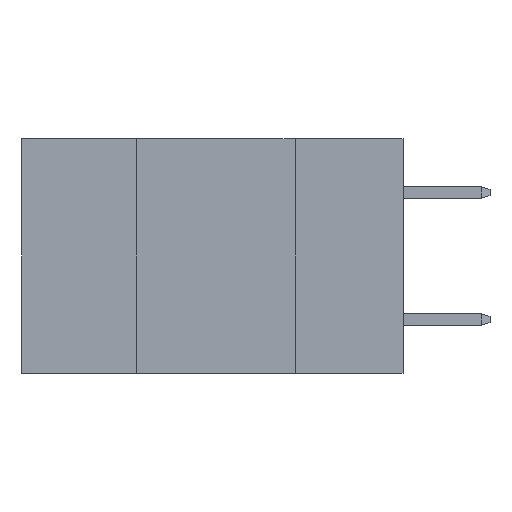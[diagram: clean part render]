
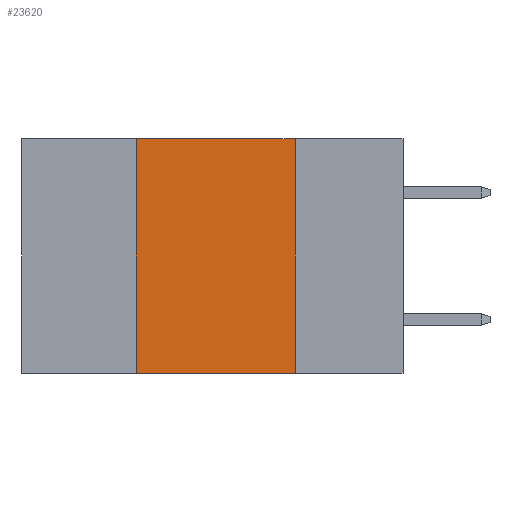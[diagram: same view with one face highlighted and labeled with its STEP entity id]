
A CAD part, left-side view. The second image highlights one B-rep face of the part: STEP entity #23620.
In plain terms, the highlighted planar face has unit normal (-1, 0, 0).
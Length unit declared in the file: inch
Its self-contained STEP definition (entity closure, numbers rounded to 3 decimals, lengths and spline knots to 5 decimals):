
#1171 = DIRECTION ( 'NONE',  ( 0., 0., -1. ) ) ;
#1890 = CARTESIAN_POINT ( 'NONE',  ( 0., 0.17, 0. ) ) ;
#1953 = CARTESIAN_POINT ( 'NONE',  ( 0., 0.6, 0. ) ) ;
#2486 = EDGE_CURVE ( 'NONE', #7120, #14501, #8160, .T. ) ;
#3220 = LINE ( 'NONE', #17928, #13040 ) ;
#3814 = CARTESIAN_POINT ( 'NONE',  ( 0., 0.42, 0. ) ) ;
#4057 = DIRECTION ( 'NONE',  ( 0., -1., 0. ) ) ;
#4792 = PLANE ( 'NONE',  #8637 ) ;
#4900 = CARTESIAN_POINT ( 'NONE',  ( 0., 0.6, 0. ) ) ;
#5756 = LINE ( 'NONE', #1890, #13366 ) ;
#6649 = EDGE_LOOP ( 'NONE', ( #21218, #14954, #16603, #20751 ) ) ;
#7120 = VERTEX_POINT ( 'NONE', #22613 ) ;
#8160 = LINE ( 'NONE', #10052, #16200 ) ;
#8206 = EDGE_CURVE ( 'NONE', #14170, #14501, #5756, .T. ) ;
#8637 = AXIS2_PLACEMENT_3D ( 'NONE', #4900, #18247, #1171 ) ;
#10052 = CARTESIAN_POINT ( 'NONE',  ( 0., 0.6, -0.37 ) ) ;
#10071 = CARTESIAN_POINT ( 'NONE',  ( 0., 0.17, -0.37 ) ) ;
#10818 = EDGE_CURVE ( 'NONE', #7120, #22752, #3220, .T. ) ;
#11164 = DIRECTION ( 'NONE',  ( 0., 0., -1. ) ) ;
#13040 = VECTOR ( 'NONE', #23907, 39.37008 ) ;
#13366 = VECTOR ( 'NONE', #11164, 39.37008 ) ;
#14170 = VERTEX_POINT ( 'NONE', #23656 ) ;
#14501 = VERTEX_POINT ( 'NONE', #10071 ) ;
#14954 = ORIENTED_EDGE ( 'NONE', *, *, #24196, .F. ) ;
#16200 = VECTOR ( 'NONE', #4057, 39.37008 ) ;
#16603 = ORIENTED_EDGE ( 'NONE', *, *, #10818, .F. ) ;
#17419 = DIRECTION ( 'NONE',  ( 0., -1., 0. ) ) ;
#17821 = VECTOR ( 'NONE', #17419, 39.37008 ) ;
#17928 = CARTESIAN_POINT ( 'NONE',  ( 0., 0.42, 0. ) ) ;
#18247 = DIRECTION ( 'NONE',  ( 1., 0., 0. ) ) ;
#20751 = ORIENTED_EDGE ( 'NONE', *, *, #2486, .T. ) ;
#20891 = LINE ( 'NONE', #1953, #17821 ) ;
#21218 = ORIENTED_EDGE ( 'NONE', *, *, #8206, .F. ) ;
#22613 = CARTESIAN_POINT ( 'NONE',  ( 0., 0.42, -0.37 ) ) ;
#22752 = VERTEX_POINT ( 'NONE', #3814 ) ;
#23620 = ADVANCED_FACE ( 'NONE', ( #23717 ), #4792, .F. ) ;
#23656 = CARTESIAN_POINT ( 'NONE',  ( 0., 0.17, 0. ) ) ;
#23717 = FACE_OUTER_BOUND ( 'NONE', #6649, .T. ) ;
#23907 = DIRECTION ( 'NONE',  ( 0., 0., 1. ) ) ;
#24196 = EDGE_CURVE ( 'NONE', #22752, #14170, #20891, .T. ) ;
